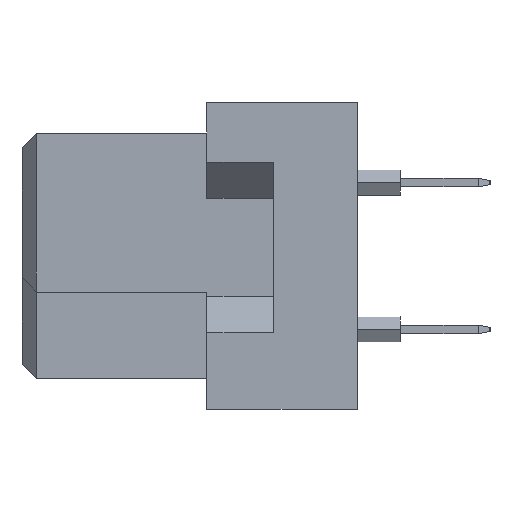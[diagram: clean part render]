
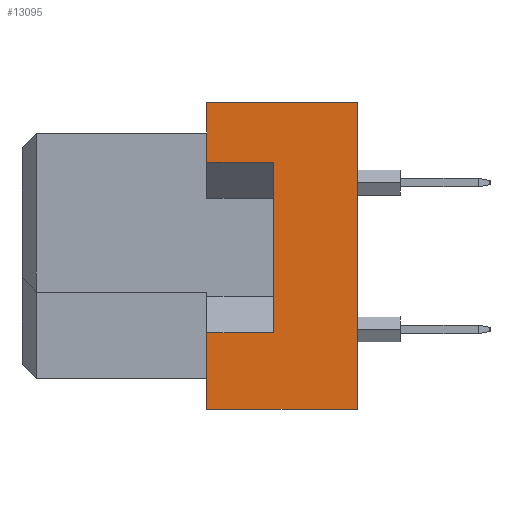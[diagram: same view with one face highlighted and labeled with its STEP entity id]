
A CAD part, left-side view. The second image highlights one B-rep face of the part: STEP entity #13095.
In plain terms, the highlighted planar face has unit normal (-1, 0, 0).
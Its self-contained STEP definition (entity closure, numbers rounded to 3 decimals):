
#1077 = VERTEX_POINT ( 'NONE', #18717 ) ;
#1126 = EDGE_CURVE ( 'NONE', #34262, #20264, #18920, .T. ) ;
#1211 = VECTOR ( 'NONE', #25146, 1000. ) ;
#1893 = CARTESIAN_POINT ( 'NONE',  ( -47.5, -11.6, 5.3 ) ) ;
#2060 = DIRECTION ( 'NONE',  ( 0., 1., 0. ) ) ;
#2239 = DIRECTION ( 'NONE',  ( 0., 0., 1. ) ) ;
#3546 = EDGE_CURVE ( 'NONE', #34262, #16978, #13692, .T. ) ;
#4550 = VECTOR ( 'NONE', #9406, 1000. ) ;
#5363 = CARTESIAN_POINT ( 'NONE',  ( -47.5, -6.4, 3.25 ) ) ;
#6165 = EDGE_CURVE ( 'NONE', #22296, #1077, #12513, .T. ) ;
#7368 = VERTEX_POINT ( 'NONE', #15958 ) ;
#7729 = EDGE_CURVE ( 'NONE', #20264, #7368, #12864, .T. ) ;
#8694 = CARTESIAN_POINT ( 'NONE',  ( -47.5, -6.4, -5.3 ) ) ;
#8699 = DIRECTION ( 'NONE',  ( -1., 0., 0. ) ) ;
#9324 = CARTESIAN_POINT ( 'NONE',  ( -47.5, -11.6, -5.3 ) ) ;
#9406 = DIRECTION ( 'NONE',  ( 0., 1., 0. ) ) ;
#10316 = LINE ( 'NONE', #22656, #28196 ) ;
#10649 = ORIENTED_EDGE ( 'NONE', *, *, #17942, .T. ) ;
#12257 = DIRECTION ( 'NONE',  ( 0., 1., 0. ) ) ;
#12513 = LINE ( 'NONE', #24854, #13799 ) ;
#12797 = ORIENTED_EDGE ( 'NONE', *, *, #3546, .T. ) ;
#12864 = LINE ( 'NONE', #28246, #28147 ) ;
#13095 = ADVANCED_FACE ( 'NONE', ( #23502 ), #29762, .T. ) ;
#13692 = LINE ( 'NONE', #17136, #36994 ) ;
#13799 = VECTOR ( 'NONE', #27889, 1000. ) ;
#15958 = CARTESIAN_POINT ( 'NONE',  ( -47.5, -6.4, -2.65 ) ) ;
#16135 = VECTOR ( 'NONE', #12257, 1000. ) ;
#16978 = VERTEX_POINT ( 'NONE', #1893 ) ;
#17136 = CARTESIAN_POINT ( 'NONE',  ( -47.5, -11.6, 5.3 ) ) ;
#17942 = EDGE_CURVE ( 'NONE', #16978, #1077, #39960, .T. ) ;
#18179 = ORIENTED_EDGE ( 'NONE', *, *, #1126, .F. ) ;
#18717 = CARTESIAN_POINT ( 'NONE',  ( -47.5, -6.4, 5.3 ) ) ;
#18920 = LINE ( 'NONE', #39748, #4550 ) ;
#19529 = CARTESIAN_POINT ( 'NONE',  ( -47.5, -8.7, -2.65 ) ) ;
#19638 = DIRECTION ( 'NONE',  ( 0., 0., 1. ) ) ;
#20264 = VERTEX_POINT ( 'NONE', #8694 ) ;
#20393 = VERTEX_POINT ( 'NONE', #33196 ) ;
#20863 = CARTESIAN_POINT ( 'NONE',  ( -47.5, -11.6, 5.3 ) ) ;
#21934 = VECTOR ( 'NONE', #2060, 1000. ) ;
#22248 = ORIENTED_EDGE ( 'NONE', *, *, #30450, .F. ) ;
#22296 = VERTEX_POINT ( 'NONE', #5363 ) ;
#22656 = CARTESIAN_POINT ( 'NONE',  ( -47.5, -8.7, -2.65 ) ) ;
#23009 = EDGE_LOOP ( 'NONE', ( #36354, #33924, #18179, #12797, #10649, #29269, #22248, #32846 ) ) ;
#23502 = FACE_OUTER_BOUND ( 'NONE', #23009, .T. ) ;
#24854 = CARTESIAN_POINT ( 'NONE',  ( -47.5, -6.4, -5.3 ) ) ;
#25146 = DIRECTION ( 'NONE',  ( 0., 1., 0. ) ) ;
#25207 = DIRECTION ( 'NONE',  ( 0., 0., 1. ) ) ;
#26037 = DIRECTION ( 'NONE',  ( 0., 0., 1. ) ) ;
#26327 = AXIS2_PLACEMENT_3D ( 'NONE', #20863, #8699, #2239 ) ;
#27314 = EDGE_CURVE ( 'NONE', #38913, #20393, #10316, .T. ) ;
#27347 = LINE ( 'NONE', #29992, #21934 ) ;
#27780 = LINE ( 'NONE', #34062, #1211 ) ;
#27889 = DIRECTION ( 'NONE',  ( 0., 0., 1. ) ) ;
#28147 = VECTOR ( 'NONE', #25207, 1000. ) ;
#28196 = VECTOR ( 'NONE', #19638, 1000. ) ;
#28246 = CARTESIAN_POINT ( 'NONE',  ( -47.5, -6.4, -5.3 ) ) ;
#29269 = ORIENTED_EDGE ( 'NONE', *, *, #6165, .F. ) ;
#29762 = PLANE ( 'NONE',  #26327 ) ;
#29992 = CARTESIAN_POINT ( 'NONE',  ( -47.5, -8.7, 3.25 ) ) ;
#30223 = EDGE_CURVE ( 'NONE', #38913, #7368, #27780, .T. ) ;
#30450 = EDGE_CURVE ( 'NONE', #20393, #22296, #27347, .T. ) ;
#31074 = CARTESIAN_POINT ( 'NONE',  ( -47.5, -11.6, 5.3 ) ) ;
#32846 = ORIENTED_EDGE ( 'NONE', *, *, #27314, .F. ) ;
#33196 = CARTESIAN_POINT ( 'NONE',  ( -47.5, -8.7, 3.25 ) ) ;
#33924 = ORIENTED_EDGE ( 'NONE', *, *, #7729, .F. ) ;
#34062 = CARTESIAN_POINT ( 'NONE',  ( -47.5, -8.7, -2.65 ) ) ;
#34262 = VERTEX_POINT ( 'NONE', #9324 ) ;
#36354 = ORIENTED_EDGE ( 'NONE', *, *, #30223, .T. ) ;
#36994 = VECTOR ( 'NONE', #26037, 1000. ) ;
#38913 = VERTEX_POINT ( 'NONE', #19529 ) ;
#39748 = CARTESIAN_POINT ( 'NONE',  ( -47.5, -11.6, -5.3 ) ) ;
#39960 = LINE ( 'NONE', #31074, #16135 ) ;
